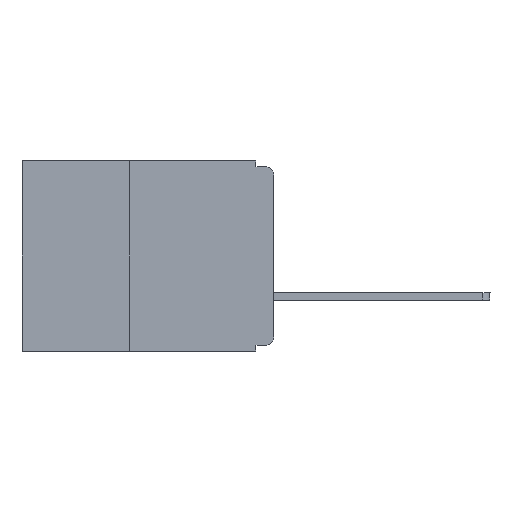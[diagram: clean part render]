
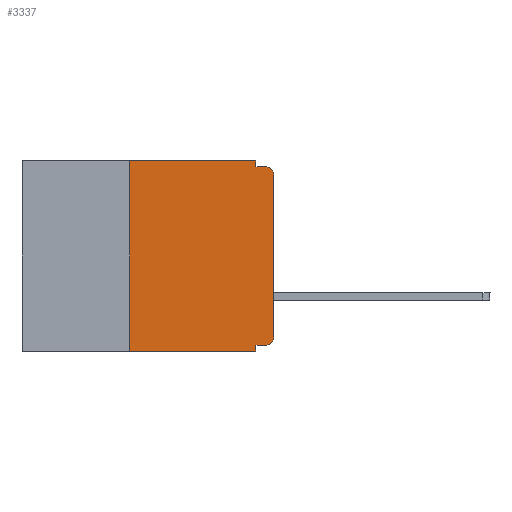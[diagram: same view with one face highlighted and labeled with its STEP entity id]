
A CAD part, left-side view. The second image highlights one B-rep face of the part: STEP entity #3337.
In plain terms, the highlighted planar face has unit normal (-1, 0, 0).
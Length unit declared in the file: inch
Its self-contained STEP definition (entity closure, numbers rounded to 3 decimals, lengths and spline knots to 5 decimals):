
#579 = CARTESIAN_POINT ( 'NONE',  ( 0., 0.031, -0.32 ) ) ;
#609 = ORIENTED_EDGE ( 'NONE', *, *, #9402, .F. ) ;
#730 = VERTEX_POINT ( 'NONE', #2237 ) ;
#750 = CARTESIAN_POINT ( 'NONE',  ( 0., 0.031, -0.33 ) ) ;
#841 = DIRECTION ( 'NONE',  ( 0., 0., -1. ) ) ;
#903 = EDGE_CURVE ( 'NONE', #730, #1640, #5932, .T. ) ;
#950 = CARTESIAN_POINT ( 'NONE',  ( 0., 0.25, -0.33 ) ) ;
#952 = AXIS2_PLACEMENT_3D ( 'NONE', #8537, #3108, #12915 ) ;
#1014 = CARTESIAN_POINT ( 'NONE',  ( 0., 0.015, -0.305 ) ) ;
#1191 = CARTESIAN_POINT ( 'NONE',  ( 0., 0., -0.305 ) ) ;
#1309 = DIRECTION ( 'NONE',  ( 0., 1., 0. ) ) ;
#1550 = CARTESIAN_POINT ( 'NONE',  ( 0., 0.031, 0. ) ) ;
#1640 = VERTEX_POINT ( 'NONE', #2115 ) ;
#1728 = DIRECTION ( 'NONE',  ( 0., -1., 0. ) ) ;
#1985 = PLANE ( 'NONE',  #952 ) ;
#2115 = CARTESIAN_POINT ( 'NONE',  ( 0., 0.015, -0.01 ) ) ;
#2237 = CARTESIAN_POINT ( 'NONE',  ( 0., 0.031, -0.01 ) ) ;
#2319 = CARTESIAN_POINT ( 'NONE',  ( 0., 0., -0.32 ) ) ;
#2469 = CARTESIAN_POINT ( 'NONE',  ( 0., 0.25, 0. ) ) ;
#2657 = EDGE_CURVE ( 'NONE', #3621, #2815, #9791, .T. ) ;
#2721 = VECTOR ( 'NONE', #12100, 39.37008 ) ;
#2815 = VERTEX_POINT ( 'NONE', #1191 ) ;
#2981 = CARTESIAN_POINT ( 'NONE',  ( 0., 0.437, 0. ) ) ;
#3033 = ORIENTED_EDGE ( 'NONE', *, *, #903, .F. ) ;
#3057 = EDGE_LOOP ( 'NONE', ( #7783, #11263, #3033, #13268, #609, #13640, #12277, #4449, #6421, #8896 ) ) ;
#3108 = DIRECTION ( 'NONE',  ( 1., 0., 0. ) ) ;
#3337 = ADVANCED_FACE ( 'NONE', ( #5404 ), #1985, .F. ) ;
#3568 = CARTESIAN_POINT ( 'NONE',  ( 0., 0., 0. ) ) ;
#3621 = VERTEX_POINT ( 'NONE', #12339 ) ;
#3795 = VECTOR ( 'NONE', #5666, 39.37008 ) ;
#3919 = DIRECTION ( 'NONE',  ( 0., 0., 1. ) ) ;
#4089 = VECTOR ( 'NONE', #1728, 39.37008 ) ;
#4449 = ORIENTED_EDGE ( 'NONE', *, *, #12222, .F. ) ;
#4946 = VERTEX_POINT ( 'NONE', #1550 ) ;
#5341 = VERTEX_POINT ( 'NONE', #2469 ) ;
#5404 = FACE_OUTER_BOUND ( 'NONE', #3057, .T. ) ;
#5621 = VECTOR ( 'NONE', #3919, 39.37008 ) ;
#5666 = DIRECTION ( 'NONE',  ( 0., 0., -1. ) ) ;
#5932 = LINE ( 'NONE', #12499, #4089 ) ;
#6207 = LINE ( 'NONE', #11605, #12296 ) ;
#6421 = ORIENTED_EDGE ( 'NONE', *, *, #11061, .F. ) ;
#6528 = LINE ( 'NONE', #3568, #2721 ) ;
#6535 = EDGE_CURVE ( 'NONE', #2815, #6724, #6528, .T. ) ;
#6724 = VERTEX_POINT ( 'NONE', #9593 ) ;
#6801 = CARTESIAN_POINT ( 'NONE',  ( 0., 0.031, 0. ) ) ;
#7238 = DIRECTION ( 'NONE',  ( 0., -1., 0. ) ) ;
#7522 = CIRCLE ( 'NONE', #9683, 0.015 ) ;
#7651 = LINE ( 'NONE', #2981, #9198 ) ;
#7656 = LINE ( 'NONE', #6801, #3795 ) ;
#7783 = ORIENTED_EDGE ( 'NONE', *, *, #6535, .T. ) ;
#8537 = CARTESIAN_POINT ( 'NONE',  ( 0., 0.437, 0. ) ) ;
#8749 = VECTOR ( 'NONE', #1309, 39.37008 ) ;
#8870 = LINE ( 'NONE', #11157, #5621 ) ;
#8896 = ORIENTED_EDGE ( 'NONE', *, *, #2657, .T. ) ;
#9065 = LINE ( 'NONE', #750, #13095 ) ;
#9075 = DIRECTION ( 'NONE',  ( -1., 0., 0. ) ) ;
#9141 = AXIS2_PLACEMENT_3D ( 'NONE', #1014, #11592, #10626 ) ;
#9198 = VECTOR ( 'NONE', #7238, 39.37008 ) ;
#9398 = DIRECTION ( 'NONE',  ( 0., -1., 0. ) ) ;
#9402 = EDGE_CURVE ( 'NONE', #5341, #4946, #7651, .T. ) ;
#9593 = CARTESIAN_POINT ( 'NONE',  ( 0., 0., -0.025 ) ) ;
#9683 = AXIS2_PLACEMENT_3D ( 'NONE', #12460, #9075, #11378 ) ;
#9791 = CIRCLE ( 'NONE', #9141, 0.015 ) ;
#10626 = DIRECTION ( 'NONE',  ( 0., 0., -1. ) ) ;
#10756 = EDGE_CURVE ( 'NONE', #13112, #11332, #6207, .T. ) ;
#11061 = EDGE_CURVE ( 'NONE', #3621, #11110, #13803, .T. ) ;
#11110 = VERTEX_POINT ( 'NONE', #579 ) ;
#11157 = CARTESIAN_POINT ( 'NONE',  ( 0., 0.25, -0.33 ) ) ;
#11263 = ORIENTED_EDGE ( 'NONE', *, *, #11993, .T. ) ;
#11332 = VERTEX_POINT ( 'NONE', #13700 ) ;
#11378 = DIRECTION ( 'NONE',  ( 0., 0., -1. ) ) ;
#11592 = DIRECTION ( 'NONE',  ( -1., 0., 0. ) ) ;
#11605 = CARTESIAN_POINT ( 'NONE',  ( 0., 0.437, -0.33 ) ) ;
#11993 = EDGE_CURVE ( 'NONE', #6724, #1640, #7522, .T. ) ;
#12100 = DIRECTION ( 'NONE',  ( 0., 0., 1. ) ) ;
#12222 = EDGE_CURVE ( 'NONE', #11110, #11332, #9065, .T. ) ;
#12277 = ORIENTED_EDGE ( 'NONE', *, *, #10756, .T. ) ;
#12296 = VECTOR ( 'NONE', #9398, 39.37008 ) ;
#12339 = CARTESIAN_POINT ( 'NONE',  ( 0., 0.015, -0.32 ) ) ;
#12460 = CARTESIAN_POINT ( 'NONE',  ( 0., 0.015, -0.025 ) ) ;
#12499 = CARTESIAN_POINT ( 'NONE',  ( 0., 0., -0.01 ) ) ;
#12915 = DIRECTION ( 'NONE',  ( 0., 0., -1. ) ) ;
#13095 = VECTOR ( 'NONE', #841, 39.37008 ) ;
#13112 = VERTEX_POINT ( 'NONE', #950 ) ;
#13268 = ORIENTED_EDGE ( 'NONE', *, *, #13659, .F. ) ;
#13271 = EDGE_CURVE ( 'NONE', #13112, #5341, #8870, .T. ) ;
#13640 = ORIENTED_EDGE ( 'NONE', *, *, #13271, .F. ) ;
#13659 = EDGE_CURVE ( 'NONE', #4946, #730, #7656, .T. ) ;
#13700 = CARTESIAN_POINT ( 'NONE',  ( 0., 0.031, -0.33 ) ) ;
#13803 = LINE ( 'NONE', #2319, #8749 ) ;
